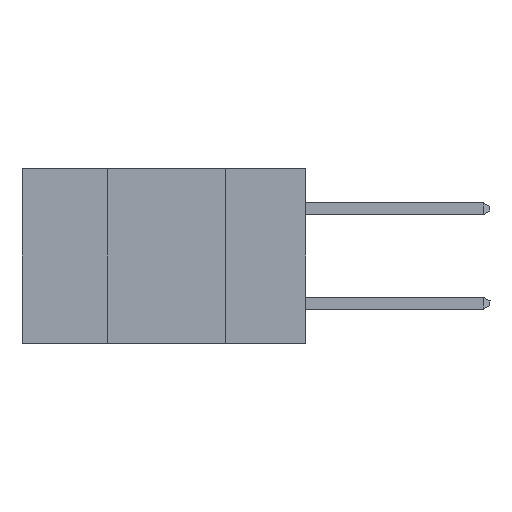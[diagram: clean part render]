
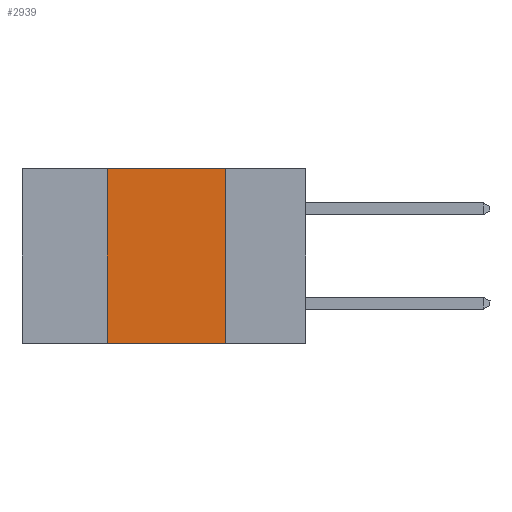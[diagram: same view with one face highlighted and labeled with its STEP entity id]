
A CAD part, left-side view. The second image highlights one B-rep face of the part: STEP entity #2939.
In plain terms, the highlighted planar face has unit normal (-1, 0, 0).
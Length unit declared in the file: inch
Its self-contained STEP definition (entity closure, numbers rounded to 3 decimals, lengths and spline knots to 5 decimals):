
#216 = DIRECTION ( 'NONE',  ( 0., -1., 0. ) ) ;
#307 = DIRECTION ( 'NONE',  ( 0., 0., -1. ) ) ;
#442 = ORIENTED_EDGE ( 'NONE', *, *, #12047, .F. ) ;
#639 = LINE ( 'NONE', #2666, #5956 ) ;
#1359 = ORIENTED_EDGE ( 'NONE', *, *, #14855, .F. ) ;
#1651 = CARTESIAN_POINT ( 'NONE',  ( 0., 0.17, -0.37 ) ) ;
#2014 = DIRECTION ( 'NONE',  ( 0., 0., 1. ) ) ;
#2297 = LINE ( 'NONE', #10401, #6349 ) ;
#2584 = VERTEX_POINT ( 'NONE', #1651 ) ;
#2666 = CARTESIAN_POINT ( 'NONE',  ( 0., 0.17, 0. ) ) ;
#2766 = CARTESIAN_POINT ( 'NONE',  ( 0., 0.42, -0.37 ) ) ;
#2831 = ORIENTED_EDGE ( 'NONE', *, *, #15149, .F. ) ;
#2939 = ADVANCED_FACE ( 'NONE', ( #7402 ), #14342, .F. ) ;
#3668 = DIRECTION ( 'NONE',  ( 0., 0., -1. ) ) ;
#4189 = EDGE_CURVE ( 'NONE', #15179, #2584, #14065, .T. ) ;
#4714 = VECTOR ( 'NONE', #12154, 39.37008 ) ;
#5845 = VECTOR ( 'NONE', #216, 39.37008 ) ;
#5956 = VECTOR ( 'NONE', #3668, 39.37008 ) ;
#6349 = VECTOR ( 'NONE', #2014, 39.37008 ) ;
#7402 = FACE_OUTER_BOUND ( 'NONE', #13997, .T. ) ;
#7538 = LINE ( 'NONE', #14252, #5845 ) ;
#9961 = CARTESIAN_POINT ( 'NONE',  ( 0., 0.6, -0.37 ) ) ;
#10401 = CARTESIAN_POINT ( 'NONE',  ( 0., 0.42, 0. ) ) ;
#10577 = VERTEX_POINT ( 'NONE', #12456 ) ;
#10766 = ORIENTED_EDGE ( 'NONE', *, *, #4189, .T. ) ;
#12039 = CARTESIAN_POINT ( 'NONE',  ( 0., 0.6, 0. ) ) ;
#12047 = EDGE_CURVE ( 'NONE', #10577, #12721, #7538, .T. ) ;
#12154 = DIRECTION ( 'NONE',  ( 0., -1., 0. ) ) ;
#12456 = CARTESIAN_POINT ( 'NONE',  ( 0., 0.42, 0. ) ) ;
#12721 = VERTEX_POINT ( 'NONE', #14749 ) ;
#12827 = AXIS2_PLACEMENT_3D ( 'NONE', #12039, #14394, #307 ) ;
#13997 = EDGE_LOOP ( 'NONE', ( #2831, #442, #1359, #10766 ) ) ;
#14065 = LINE ( 'NONE', #9961, #4714 ) ;
#14252 = CARTESIAN_POINT ( 'NONE',  ( 0., 0.6, 0. ) ) ;
#14342 = PLANE ( 'NONE',  #12827 ) ;
#14394 = DIRECTION ( 'NONE',  ( 1., 0., 0. ) ) ;
#14749 = CARTESIAN_POINT ( 'NONE',  ( 0., 0.17, 0. ) ) ;
#14855 = EDGE_CURVE ( 'NONE', #15179, #10577, #2297, .T. ) ;
#15149 = EDGE_CURVE ( 'NONE', #12721, #2584, #639, .T. ) ;
#15179 = VERTEX_POINT ( 'NONE', #2766 ) ;
